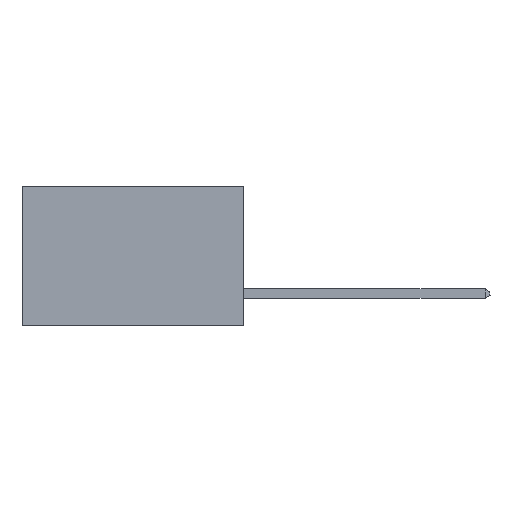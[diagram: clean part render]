
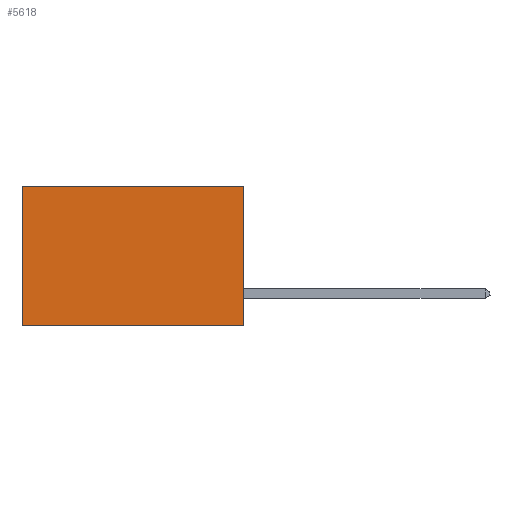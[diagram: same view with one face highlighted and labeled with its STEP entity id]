
A CAD part, left-side view. The second image highlights one B-rep face of the part: STEP entity #5618.
In plain terms, the highlighted planar face has unit normal (-1, 0, 0).
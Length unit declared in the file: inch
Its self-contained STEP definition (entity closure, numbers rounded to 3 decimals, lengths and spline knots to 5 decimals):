
#1 = DIRECTION ( 'NONE',  ( 0., 0., -1. ) ) ;
#1279 = CARTESIAN_POINT ( 'NONE',  ( 0.277, 0., 0. ) ) ;
#2196 = AXIS2_PLACEMENT_3D ( 'NONE', #5796, #5619, #5588 ) ;
#3092 = DIRECTION ( 'NONE',  ( 0., 1., 0. ) ) ;
#3438 = CARTESIAN_POINT ( 'NONE',  ( 0.277, 0., 0. ) ) ;
#5588 = DIRECTION ( 'NONE',  ( 0., 0., -1. ) ) ;
#5618 = ADVANCED_FACE ( 'NONE', ( #12302 ), #5649, .F. ) ;
#5619 = DIRECTION ( 'NONE',  ( 1., 0., 0. ) ) ;
#5649 = PLANE ( 'NONE',  #2196 ) ;
#5796 = CARTESIAN_POINT ( 'NONE',  ( 0.277, 0., -0.37 ) ) ;
#5820 = VERTEX_POINT ( 'NONE', #1279 ) ;
#6548 = CARTESIAN_POINT ( 'NONE',  ( 0.277, 0.59, 0. ) ) ;
#6682 = EDGE_LOOP ( 'NONE', ( #26539, #23455, #24554, #14549 ) ) ;
#8463 = VECTOR ( 'NONE', #21161, 39.37008 ) ;
#9282 = CARTESIAN_POINT ( 'NONE',  ( 0.277, 0.59, -0.37 ) ) ;
#9739 = VECTOR ( 'NONE', #3092, 39.37008 ) ;
#9779 = EDGE_CURVE ( 'NONE', #5820, #11915, #20938, .T. ) ;
#10645 = CARTESIAN_POINT ( 'NONE',  ( 0.277, 0., -0.37 ) ) ;
#11724 = VERTEX_POINT ( 'NONE', #22640 ) ;
#11915 = VERTEX_POINT ( 'NONE', #6548 ) ;
#12302 = FACE_OUTER_BOUND ( 'NONE', #6682, .T. ) ;
#13667 = LINE ( 'NONE', #10645, #19933 ) ;
#14064 = LINE ( 'NONE', #23235, #24509 ) ;
#14549 = ORIENTED_EDGE ( 'NONE', *, *, #9779, .T. ) ;
#14758 = LINE ( 'NONE', #14822, #8463 ) ;
#14822 = CARTESIAN_POINT ( 'NONE',  ( 0.277, 0.59, -0.37 ) ) ;
#16293 = VERTEX_POINT ( 'NONE', #9282 ) ;
#19686 = EDGE_CURVE ( 'NONE', #11915, #16293, #14758, .T. ) ;
#19688 = EDGE_CURVE ( 'NONE', #5820, #11724, #14064, .T. ) ;
#19933 = VECTOR ( 'NONE', #25273, 39.37008 ) ;
#20938 = LINE ( 'NONE', #3438, #9739 ) ;
#21161 = DIRECTION ( 'NONE',  ( 0., 0., -1. ) ) ;
#22640 = CARTESIAN_POINT ( 'NONE',  ( 0.277, 0., -0.37 ) ) ;
#23235 = CARTESIAN_POINT ( 'NONE',  ( 0.277, 0., -0.37 ) ) ;
#23455 = ORIENTED_EDGE ( 'NONE', *, *, #25180, .F. ) ;
#24509 = VECTOR ( 'NONE', #1, 39.37008 ) ;
#24554 = ORIENTED_EDGE ( 'NONE', *, *, #19688, .F. ) ;
#25180 = EDGE_CURVE ( 'NONE', #11724, #16293, #13667, .T. ) ;
#25273 = DIRECTION ( 'NONE',  ( 0., 1., 0. ) ) ;
#26539 = ORIENTED_EDGE ( 'NONE', *, *, #19686, .T. ) ;
